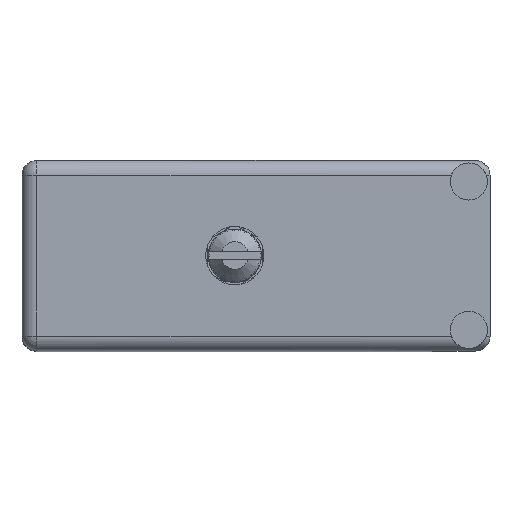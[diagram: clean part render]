
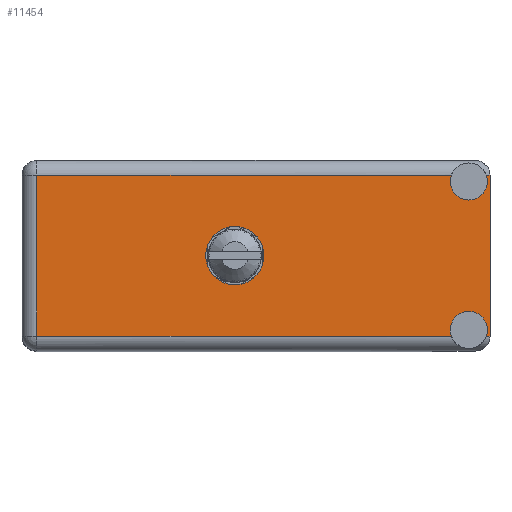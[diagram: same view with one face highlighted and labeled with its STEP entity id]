
A CAD part, top view. The second image highlights one B-rep face of the part: STEP entity #11454.
In plain terms, the highlighted face is planar.
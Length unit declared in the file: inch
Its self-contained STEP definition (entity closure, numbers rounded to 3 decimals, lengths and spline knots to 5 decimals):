
#19 = CARTESIAN_POINT ( 'NONE',  ( 0., 1.466, 0.1375 ) ) ;
#1768 = CARTESIAN_POINT ( 'NONE',  ( 1.104, 1.466, -0.2625 ) ) ;
#5424 = CARTESIAN_POINT ( 'NONE',  ( 1.02162, 1.466, -0.3795 ) ) ;
#6244 = DIRECTION ( 'NONE',  ( 0., 0., 1. ) ) ;
#6751 = ORIENTED_EDGE ( 'NONE', *, *, #95484, .T. ) ;
#7557 = LINE ( 'NONE', #100586, #58570 ) ;
#7888 = AXIS2_PLACEMENT_3D ( 'NONE', #53707, #45857, #54061 ) ;
#7948 = CARTESIAN_POINT ( 'NONE',  ( 1.104, 1.466, -0.35 ) ) ;
#8112 = ORIENTED_EDGE ( 'NONE', *, *, #23881, .F. ) ;
#8410 = ORIENTED_EDGE ( 'NONE', *, *, #51945, .F. ) ;
#8699 = DIRECTION ( 'NONE',  ( 1., 0., 0. ) ) ;
#11333 = LINE ( 'NONE', #12389, #86542 ) ;
#11454 = ADVANCED_FACE ( 'NONE', ( #18374, #52892 ), #102377, .T. ) ;
#12389 = CARTESIAN_POINT ( 'NONE',  ( -0.934, 1.466, -0.4495 ) ) ;
#13451 = DIRECTION ( 'NONE',  ( 0., 0., 1. ) ) ;
#15047 = AXIS2_PLACEMENT_3D ( 'NONE', #70789, #38675, #6244 ) ;
#15142 = ORIENTED_EDGE ( 'NONE', *, *, #49768, .F. ) ;
#17273 = EDGE_CURVE ( 'NONE', #77101, #92504, #57249, .T. ) ;
#18117 = CARTESIAN_POINT ( 'NONE',  ( 0., 1.466, 0. ) ) ;
#18345 = CARTESIAN_POINT ( 'NONE',  ( 0., 1.466, 0. ) ) ;
#18374 = FACE_BOUND ( 'NONE', #74845, .T. ) ;
#18834 = CIRCLE ( 'NONE', #38525, 0.0875 ) ;
#20025 = VERTEX_POINT ( 'NONE', #1768 ) ;
#20627 = DIRECTION ( 'NONE',  ( 0., 0., 1. ) ) ;
#20974 = ORIENTED_EDGE ( 'NONE', *, *, #59909, .F. ) ;
#23881 = EDGE_CURVE ( 'NONE', #77101, #20025, #67751, .T. ) ;
#24368 = DIRECTION ( 'NONE',  ( 0., 1., 0. ) ) ;
#24407 = CARTESIAN_POINT ( 'NONE',  ( 1.204, 1.466, 0.3795 ) ) ;
#25550 = ORIENTED_EDGE ( 'NONE', *, *, #17273, .T. ) ;
#25975 = DIRECTION ( 'NONE',  ( -1., 0., 0. ) ) ;
#26121 = VERTEX_POINT ( 'NONE', #67019 ) ;
#27195 = VERTEX_POINT ( 'NONE', #19 ) ;
#27885 = VECTOR ( 'NONE', #25975, 39.37008 ) ;
#28498 = VERTEX_POINT ( 'NONE', #74216 ) ;
#29667 = EDGE_CURVE ( 'NONE', #28498, #88369, #37652, .T. ) ;
#29865 = EDGE_LOOP ( 'NONE', ( #6751, #52779, #20974, #38970, #15142, #80652, #52881, #8112, #25550, #47896 ) ) ;
#31748 = EDGE_CURVE ( 'NONE', #27195, #38188, #37814, .T. ) ;
#34383 = DIRECTION ( 'NONE',  ( 0., 0., 1. ) ) ;
#34769 = CARTESIAN_POINT ( 'NONE',  ( 1.204, 1.466, 0.3795 ) ) ;
#35712 = CIRCLE ( 'NONE', #64779, 0.0875 ) ;
#35922 = CARTESIAN_POINT ( 'NONE',  ( 1.104, 1.466, 0.2625 ) ) ;
#37652 = LINE ( 'NONE', #34769, #100012 ) ;
#37814 = CIRCLE ( 'NONE', #48600, 0.1375 ) ;
#37932 = EDGE_CURVE ( 'NONE', #91673, #94844, #35712, .T. ) ;
#38188 = VERTEX_POINT ( 'NONE', #92115 ) ;
#38426 = CARTESIAN_POINT ( 'NONE',  ( 1.104, 1.466, 0.35 ) ) ;
#38525 = AXIS2_PLACEMENT_3D ( 'NONE', #7948, #24368, #65297 ) ;
#38675 = DIRECTION ( 'NONE',  ( 0., 1., 0. ) ) ;
#38970 = ORIENTED_EDGE ( 'NONE', *, *, #29667, .T. ) ;
#39237 = VECTOR ( 'NONE', #90136, 39.37008 ) ;
#40460 = DIRECTION ( 'NONE',  ( 0., 1., 0. ) ) ;
#43365 = DIRECTION ( 'NONE',  ( 0., 1., 0. ) ) ;
#45857 = DIRECTION ( 'NONE',  ( 0., 1., 0. ) ) ;
#45889 = CARTESIAN_POINT ( 'NONE',  ( 1.02162, 1.466, 0.3795 ) ) ;
#47896 = ORIENTED_EDGE ( 'NONE', *, *, #102690, .T. ) ;
#48600 = AXIS2_PLACEMENT_3D ( 'NONE', #18345, #67176, #34383 ) ;
#48856 = CARTESIAN_POINT ( 'NONE',  ( 1.204, 1.466, 0.4495 ) ) ;
#49768 = EDGE_CURVE ( 'NONE', #80369, #88369, #88889, .T. ) ;
#50528 = DIRECTION ( 'NONE',  ( -1., 0., 0. ) ) ;
#51576 = DIRECTION ( 'NONE',  ( 0., 0., 1. ) ) ;
#51945 = EDGE_CURVE ( 'NONE', #38188, #27195, #97679, .T. ) ;
#52779 = ORIENTED_EDGE ( 'NONE', *, *, #37932, .F. ) ;
#52881 = ORIENTED_EDGE ( 'NONE', *, *, #72871, .F. ) ;
#52892 = FACE_OUTER_BOUND ( 'NONE', #29865, .T. ) ;
#53707 = CARTESIAN_POINT ( 'NONE',  ( -1.004, 1.466, -0.4495 ) ) ;
#54061 = DIRECTION ( 'NONE',  ( -1., 0., 0. ) ) ;
#56135 = VERTEX_POINT ( 'NONE', #67989 ) ;
#56477 = DIRECTION ( 'NONE',  ( 0., 0., 1. ) ) ;
#57249 = LINE ( 'NONE', #100265, #27885 ) ;
#58570 = VECTOR ( 'NONE', #50528, 39.37008 ) ;
#59909 = EDGE_CURVE ( 'NONE', #28498, #91673, #90448, .T. ) ;
#64779 = AXIS2_PLACEMENT_3D ( 'NONE', #38426, #86519, #20627 ) ;
#65297 = DIRECTION ( 'NONE',  ( 0., 0., 1. ) ) ;
#67019 = CARTESIAN_POINT ( 'NONE',  ( 1.18638, 1.466, -0.3795 ) ) ;
#67176 = DIRECTION ( 'NONE',  ( 0., 1., 0. ) ) ;
#67310 = AXIS2_PLACEMENT_3D ( 'NONE', #87099, #40460, #56477 ) ;
#67751 = CIRCLE ( 'NONE', #15047, 0.0875 ) ;
#67989 = CARTESIAN_POINT ( 'NONE',  ( -0.934, 1.466, 0.3795 ) ) ;
#70789 = CARTESIAN_POINT ( 'NONE',  ( 1.104, 1.466, -0.35 ) ) ;
#72871 = EDGE_CURVE ( 'NONE', #20025, #26121, #18834, .T. ) ;
#74216 = CARTESIAN_POINT ( 'NONE',  ( 1.18638, 1.466, 0.3795 ) ) ;
#74845 = EDGE_LOOP ( 'NONE', ( #91084, #8410 ) ) ;
#77101 = VERTEX_POINT ( 'NONE', #5424 ) ;
#80369 = VERTEX_POINT ( 'NONE', #98076 ) ;
#80652 = ORIENTED_EDGE ( 'NONE', *, *, #87925, .T. ) ;
#81258 = AXIS2_PLACEMENT_3D ( 'NONE', #18117, #43365, #51576 ) ;
#85302 = CARTESIAN_POINT ( 'NONE',  ( 1.204, 1.466, 0.3795 ) ) ;
#86519 = DIRECTION ( 'NONE',  ( 0., 1., 0. ) ) ;
#86542 = VECTOR ( 'NONE', #13451, 39.37008 ) ;
#87099 = CARTESIAN_POINT ( 'NONE',  ( 1.104, 1.466, 0.35 ) ) ;
#87925 = EDGE_CURVE ( 'NONE', #80369, #26121, #7557, .T. ) ;
#87990 = CARTESIAN_POINT ( 'NONE',  ( -0.934, 1.466, -0.3795 ) ) ;
#88369 = VERTEX_POINT ( 'NONE', #85302 ) ;
#88889 = LINE ( 'NONE', #48856, #39237 ) ;
#90136 = DIRECTION ( 'NONE',  ( 0., 0., 1. ) ) ;
#90448 = CIRCLE ( 'NONE', #67310, 0.0875 ) ;
#91084 = ORIENTED_EDGE ( 'NONE', *, *, #31748, .F. ) ;
#91673 = VERTEX_POINT ( 'NONE', #35922 ) ;
#92067 = DIRECTION ( 'NONE',  ( 1., 0., 0. ) ) ;
#92115 = CARTESIAN_POINT ( 'NONE',  ( 0., 1.466, -0.1375 ) ) ;
#92436 = VECTOR ( 'NONE', #8699, 39.37008 ) ;
#92504 = VERTEX_POINT ( 'NONE', #87990 ) ;
#94844 = VERTEX_POINT ( 'NONE', #45889 ) ;
#95484 = EDGE_CURVE ( 'NONE', #56135, #94844, #103781, .T. ) ;
#97679 = CIRCLE ( 'NONE', #81258, 0.1375 ) ;
#98076 = CARTESIAN_POINT ( 'NONE',  ( 1.204, 1.466, -0.3795 ) ) ;
#100012 = VECTOR ( 'NONE', #92067, 39.37008 ) ;
#100265 = CARTESIAN_POINT ( 'NONE',  ( -1.004, 1.466, -0.3795 ) ) ;
#100586 = CARTESIAN_POINT ( 'NONE',  ( -1.004, 1.466, -0.3795 ) ) ;
#102377 = PLANE ( 'NONE',  #7888 ) ;
#102690 = EDGE_CURVE ( 'NONE', #92504, #56135, #11333, .T. ) ;
#103781 = LINE ( 'NONE', #24407, #92436 ) ;
